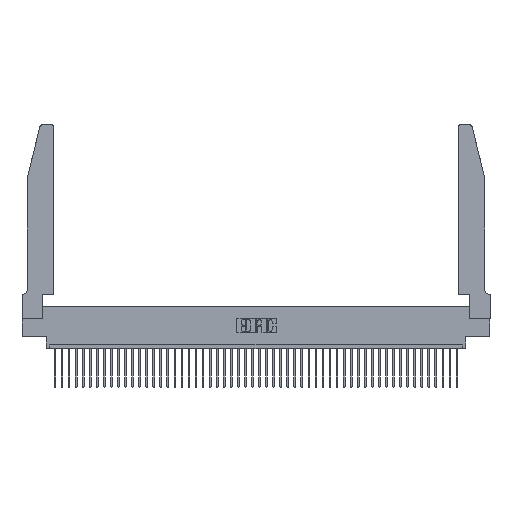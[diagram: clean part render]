
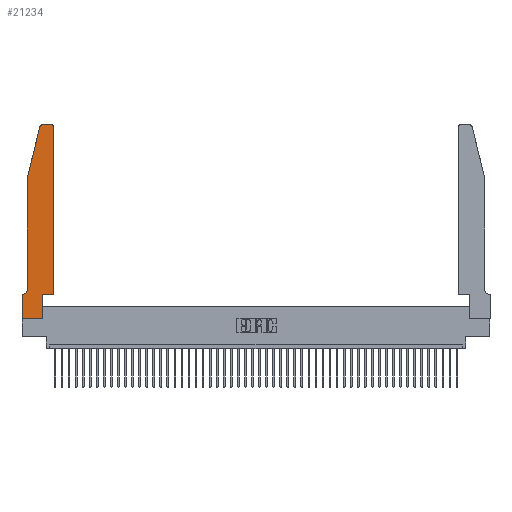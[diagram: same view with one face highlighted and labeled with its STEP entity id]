
A CAD part, top view. The second image highlights one B-rep face of the part: STEP entity #21234.
In plain terms, the highlighted planar face has unit normal (0, 0, 1).
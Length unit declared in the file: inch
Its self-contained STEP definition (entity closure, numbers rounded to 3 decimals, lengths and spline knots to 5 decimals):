
#282 = ORIENTED_EDGE ( 'NONE', *, *, #26101, .T. ) ;
#301 = LINE ( 'NONE', #26697, #1443 ) ;
#813 = DIRECTION ( 'NONE',  ( 0., -1., 0. ) ) ;
#1194 = CIRCLE ( 'NONE', #36401, 0.03 ) ;
#1443 = VECTOR ( 'NONE', #2304, 39.37008 ) ;
#1592 = EDGE_LOOP ( 'NONE', ( #19126, #11187, #14542, #43826, #2898, #27152, #6892, #3868, #40861, #282, #22545, #16924 ) ) ;
#1800 = VECTOR ( 'NONE', #8084, 39.37008 ) ;
#1892 = CARTESIAN_POINT ( 'NONE',  ( 0.0755, 0.35, 0.37 ) ) ;
#2304 = DIRECTION ( 'NONE',  ( -0.239, -0.971, 0. ) ) ;
#2898 = ORIENTED_EDGE ( 'NONE', *, *, #8899, .T. ) ;
#3243 = CARTESIAN_POINT ( 'NONE',  ( 0.0755, 0.42, 0.37 ) ) ;
#3868 = ORIENTED_EDGE ( 'NONE', *, *, #4251, .T. ) ;
#4251 = EDGE_CURVE ( 'NONE', #33673, #36329, #15220, .T. ) ;
#4318 = DIRECTION ( 'NONE',  ( 0., 0., 1. ) ) ;
#4660 = CARTESIAN_POINT ( 'NONE',  ( 0.4505, 0.35, 0.37 ) ) ;
#5175 = CARTESIAN_POINT ( 'NONE',  ( 0.25487, 2.72718, 0.37 ) ) ;
#5567 = VERTEX_POINT ( 'NONE', #6963 ) ;
#5591 = CARTESIAN_POINT ( 'NONE',  ( 0., 0., 0.37 ) ) ;
#5921 = CIRCLE ( 'NONE', #11969, 0.03 ) ;
#6585 = DIRECTION ( 'NONE',  ( 1., 0., 0. ) ) ;
#6892 = ORIENTED_EDGE ( 'NONE', *, *, #39402, .T. ) ;
#6963 = CARTESIAN_POINT ( 'NONE',  ( 0.284, 2.75, 0.37 ) ) ;
#7537 = LINE ( 'NONE', #11416, #22033 ) ;
#8036 = EDGE_CURVE ( 'NONE', #31525, #14966, #1194, .T. ) ;
#8084 = DIRECTION ( 'NONE',  ( 0., 1., 0. ) ) ;
#8398 = AXIS2_PLACEMENT_3D ( 'NONE', #28363, #4318, #14852 ) ;
#8899 = EDGE_CURVE ( 'NONE', #35918, #11115, #26343, .T. ) ;
#8998 = VERTEX_POINT ( 'NONE', #5175 ) ;
#9019 = CARTESIAN_POINT ( 'NONE',  ( 0.2605, 2.75, 0.37 ) ) ;
#9719 = VERTEX_POINT ( 'NONE', #46305 ) ;
#10076 = CARTESIAN_POINT ( 'NONE',  ( 0.0055, 0.42, 0.37 ) ) ;
#10352 = VECTOR ( 'NONE', #38343, 39.37008 ) ;
#10388 = FACE_OUTER_BOUND ( 'NONE', #1592, .T. ) ;
#10667 = DIRECTION ( 'NONE',  ( 0., 0., 1. ) ) ;
#10807 = EDGE_CURVE ( 'NONE', #14966, #5567, #35221, .T. ) ;
#11115 = VERTEX_POINT ( 'NONE', #42216 ) ;
#11187 = ORIENTED_EDGE ( 'NONE', *, *, #38650, .T. ) ;
#11215 = EDGE_CURVE ( 'NONE', #8998, #22248, #301, .T. ) ;
#11416 = CARTESIAN_POINT ( 'NONE',  ( 0., 0., 0.37 ) ) ;
#11969 = AXIS2_PLACEMENT_3D ( 'NONE', #16716, #41746, #13588 ) ;
#13264 = LINE ( 'NONE', #23130, #31154 ) ;
#13276 = CARTESIAN_POINT ( 'NONE',  ( 0.2865, 0., 0.37 ) ) ;
#13355 = EDGE_CURVE ( 'NONE', #11115, #21082, #24818, .T. ) ;
#13588 = DIRECTION ( 'NONE',  ( 1., 0., 0. ) ) ;
#14542 = ORIENTED_EDGE ( 'NONE', *, *, #11215, .T. ) ;
#14852 = DIRECTION ( 'NONE',  ( 1., 0., 0. ) ) ;
#14966 = VERTEX_POINT ( 'NONE', #15650 ) ;
#15104 = CARTESIAN_POINT ( 'NONE',  ( 0.2865, 0.35, 0.37 ) ) ;
#15220 = LINE ( 'NONE', #5591, #15789 ) ;
#15650 = CARTESIAN_POINT ( 'NONE',  ( 0.4205, 2.75, 0.37 ) ) ;
#15789 = VECTOR ( 'NONE', #30474, 39.37008 ) ;
#16703 = DIRECTION ( 'NONE',  ( 0., -1., 0. ) ) ;
#16716 = CARTESIAN_POINT ( 'NONE',  ( 0.284, 2.72, 0.37 ) ) ;
#16924 = ORIENTED_EDGE ( 'NONE', *, *, #8036, .T. ) ;
#17815 = CARTESIAN_POINT ( 'NONE',  ( 0., 0., 0.37 ) ) ;
#18165 = AXIS2_PLACEMENT_3D ( 'NONE', #10076, #35082, #34929 ) ;
#19126 = ORIENTED_EDGE ( 'NONE', *, *, #10807, .T. ) ;
#19933 = CARTESIAN_POINT ( 'NONE',  ( 0., 0.35, 0.37 ) ) ;
#21082 = VERTEX_POINT ( 'NONE', #19933 ) ;
#21234 = ADVANCED_FACE ( 'NONE', ( #10388 ), #35113, .T. ) ;
#21992 = EDGE_CURVE ( 'NONE', #36329, #9719, #44974, .T. ) ;
#22033 = VECTOR ( 'NONE', #813, 39.37008 ) ;
#22248 = VERTEX_POINT ( 'NONE', #44138 ) ;
#22545 = ORIENTED_EDGE ( 'NONE', *, *, #39842, .T. ) ;
#23130 = CARTESIAN_POINT ( 'NONE',  ( 0.4505, 0.35, 0.37 ) ) ;
#24628 = VECTOR ( 'NONE', #16703, 39.37008 ) ;
#24818 = LINE ( 'NONE', #1892, #10352 ) ;
#26077 = DIRECTION ( 'NONE',  ( 1., 0., 0. ) ) ;
#26097 = VERTEX_POINT ( 'NONE', #4660 ) ;
#26101 = EDGE_CURVE ( 'NONE', #9719, #26097, #13264, .T. ) ;
#26343 = CIRCLE ( 'NONE', #18165, 0.07 ) ;
#26697 = CARTESIAN_POINT ( 'NONE',  ( 0.0755, 2., 0.37 ) ) ;
#26979 = DIRECTION ( 'NONE',  ( -1., 0., 0. ) ) ;
#27073 = VECTOR ( 'NONE', #28605, 39.37008 ) ;
#27152 = ORIENTED_EDGE ( 'NONE', *, *, #13355, .T. ) ;
#28001 = CARTESIAN_POINT ( 'NONE',  ( 0.4205, 2.72, 0.37 ) ) ;
#28363 = CARTESIAN_POINT ( 'NONE',  ( 0., 0.35, 0.37 ) ) ;
#28605 = DIRECTION ( 'NONE',  ( 0., 1., 0. ) ) ;
#29829 = LINE ( 'NONE', #35358, #27073 ) ;
#30474 = DIRECTION ( 'NONE',  ( 1., 0., 0. ) ) ;
#31154 = VECTOR ( 'NONE', #26077, 39.37008 ) ;
#31525 = VERTEX_POINT ( 'NONE', #40228 ) ;
#33673 = VERTEX_POINT ( 'NONE', #17815 ) ;
#34646 = EDGE_CURVE ( 'NONE', #22248, #35918, #43621, .T. ) ;
#34929 = DIRECTION ( 'NONE',  ( -1., 0., 0. ) ) ;
#35082 = DIRECTION ( 'NONE',  ( 0., 0., -1. ) ) ;
#35113 = PLANE ( 'NONE',  #8398 ) ;
#35221 = LINE ( 'NONE', #9019, #42499 ) ;
#35358 = CARTESIAN_POINT ( 'NONE',  ( 0.4505, 0.35, 0.37 ) ) ;
#35918 = VERTEX_POINT ( 'NONE', #3243 ) ;
#36329 = VERTEX_POINT ( 'NONE', #13276 ) ;
#36401 = AXIS2_PLACEMENT_3D ( 'NONE', #28001, #10667, #6585 ) ;
#38343 = DIRECTION ( 'NONE',  ( -1., 0., 0. ) ) ;
#38650 = EDGE_CURVE ( 'NONE', #5567, #8998, #5921, .T. ) ;
#39402 = EDGE_CURVE ( 'NONE', #21082, #33673, #7537, .T. ) ;
#39842 = EDGE_CURVE ( 'NONE', #26097, #31525, #29829, .T. ) ;
#40228 = CARTESIAN_POINT ( 'NONE',  ( 0.4505, 2.72, 0.37 ) ) ;
#40861 = ORIENTED_EDGE ( 'NONE', *, *, #21992, .T. ) ;
#41732 = CARTESIAN_POINT ( 'NONE',  ( 0.0755, 2., 0.37 ) ) ;
#41746 = DIRECTION ( 'NONE',  ( 0., 0., 1. ) ) ;
#42216 = CARTESIAN_POINT ( 'NONE',  ( 0.0055, 0.35, 0.37 ) ) ;
#42499 = VECTOR ( 'NONE', #26979, 39.37008 ) ;
#43621 = LINE ( 'NONE', #41732, #24628 ) ;
#43826 = ORIENTED_EDGE ( 'NONE', *, *, #34646, .T. ) ;
#44138 = CARTESIAN_POINT ( 'NONE',  ( 0.0755, 2., 0.37 ) ) ;
#44974 = LINE ( 'NONE', #15104, #1800 ) ;
#46305 = CARTESIAN_POINT ( 'NONE',  ( 0.2865, 0.35, 0.37 ) ) ;
